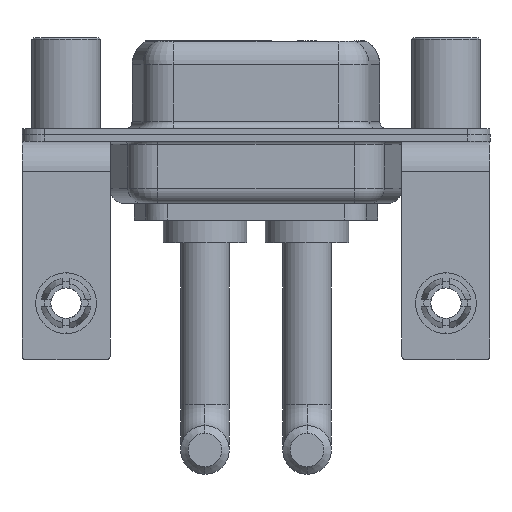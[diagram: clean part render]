
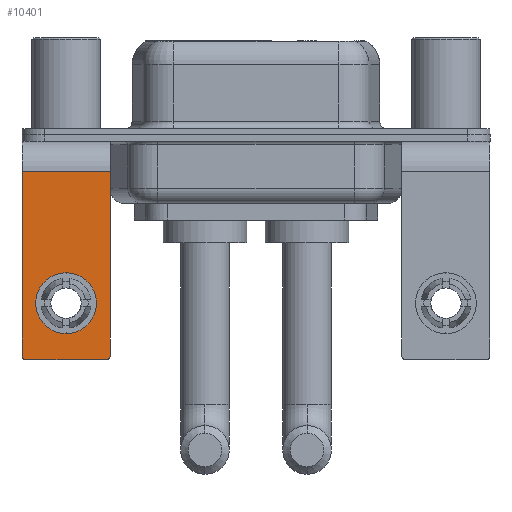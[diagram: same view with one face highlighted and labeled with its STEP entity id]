
A CAD part, front view. The second image highlights one B-rep face of the part: STEP entity #10401.
In plain terms, the highlighted planar face has unit normal (0, -1, 0).
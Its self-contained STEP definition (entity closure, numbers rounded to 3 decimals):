
#57 = CARTESIAN_POINT ( 'NONE',  ( 0., -6.25, -11.07 ) ) ;
#238 = DIRECTION ( 'NONE',  ( 0., 0., 1. ) ) ;
#415 = LINE ( 'NONE', #11838, #12715 ) ;
#627 = CARTESIAN_POINT ( 'NONE',  ( -2.9, -6.25, -2.4 ) ) ;
#634 = VERTEX_POINT ( 'NONE', #9744 ) ;
#840 = ORIENTED_EDGE ( 'NONE', *, *, #11025, .T. ) ;
#907 = VERTEX_POINT ( 'NONE', #14019 ) ;
#1452 = ORIENTED_EDGE ( 'NONE', *, *, #11088, .T. ) ;
#1684 = EDGE_CURVE ( 'NONE', #11396, #2459, #415, .T. ) ;
#1938 = VERTEX_POINT ( 'NONE', #7392 ) ;
#2459 = VERTEX_POINT ( 'NONE', #6097 ) ;
#3362 = CARTESIAN_POINT ( 'NONE',  ( -2.65, -6.25, -14.55 ) ) ;
#3517 = VECTOR ( 'NONE', #6561, 1000. ) ;
#3568 = LINE ( 'NONE', #8512, #11217 ) ;
#3751 = CARTESIAN_POINT ( 'NONE',  ( 2.9, -6.25, -14.8 ) ) ;
#3844 = EDGE_CURVE ( 'NONE', #8929, #10270, #5111, .T. ) ;
#3912 = DIRECTION ( 'NONE',  ( 0., 1., 0. ) ) ;
#3952 = CARTESIAN_POINT ( 'NONE',  ( 2.9, -6.25, -2.4 ) ) ;
#4049 = DIRECTION ( 'NONE',  ( 0., 0., 1. ) ) ;
#4340 = AXIS2_PLACEMENT_3D ( 'NONE', #5327, #14279, #4049 ) ;
#4439 = VERTEX_POINT ( 'NONE', #16140 ) ;
#4689 = AXIS2_PLACEMENT_3D ( 'NONE', #13130, #12094, #238 ) ;
#4721 = LINE ( 'NONE', #627, #5753 ) ;
#5111 = LINE ( 'NONE', #3751, #3517 ) ;
#5327 = CARTESIAN_POINT ( 'NONE',  ( 2.65, -6.25, -14.55 ) ) ;
#5480 = AXIS2_PLACEMENT_3D ( 'NONE', #3362, #13765, #10933 ) ;
#5485 = ORIENTED_EDGE ( 'NONE', *, *, #12165, .F. ) ;
#5627 = DIRECTION ( 'NONE',  ( -1., 0., 0. ) ) ;
#5642 = CARTESIAN_POINT ( 'NONE',  ( -2.65, -6.25, -14.8 ) ) ;
#5753 = VECTOR ( 'NONE', #14873, 1000. ) ;
#5783 = EDGE_LOOP ( 'NONE', ( #1452, #840, #5959, #12111, #5485, #14763 ) ) ;
#5956 = EDGE_CURVE ( 'NONE', #1938, #634, #7096, .T. ) ;
#5959 = ORIENTED_EDGE ( 'NONE', *, *, #3844, .F. ) ;
#6097 = CARTESIAN_POINT ( 'NONE',  ( -2.9, -6.25, -2.4 ) ) ;
#6231 = FACE_OUTER_BOUND ( 'NONE', #5783, .T. ) ;
#6299 = CIRCLE ( 'NONE', #5480, 0.25 ) ;
#6561 = DIRECTION ( 'NONE',  ( -1., 0., 0. ) ) ;
#7029 = CARTESIAN_POINT ( 'NONE',  ( 2.65, -6.25, -14.8 ) ) ;
#7096 = CIRCLE ( 'NONE', #16633, 2. ) ;
#7226 = ORIENTED_EDGE ( 'NONE', *, *, #13735, .T. ) ;
#7254 = DIRECTION ( 'NONE',  ( 0., 1., 0. ) ) ;
#7392 = CARTESIAN_POINT ( 'NONE',  ( 0., -6.25, -13.07 ) ) ;
#7878 = CIRCLE ( 'NONE', #4340, 0.25 ) ;
#8512 = CARTESIAN_POINT ( 'NONE',  ( 2.9, -6.25, -2.4 ) ) ;
#8772 = CIRCLE ( 'NONE', #4689, 2. ) ;
#8929 = VERTEX_POINT ( 'NONE', #7029 ) ;
#9444 = EDGE_LOOP ( 'NONE', ( #10554, #7226 ) ) ;
#9606 = EDGE_CURVE ( 'NONE', #8929, #4439, #7878, .T. ) ;
#9744 = CARTESIAN_POINT ( 'NONE',  ( 0., -6.25, -9.07 ) ) ;
#10270 = VERTEX_POINT ( 'NONE', #5642 ) ;
#10401 = ADVANCED_FACE ( 'NONE', ( #16711, #6231 ), #11512, .F. ) ;
#10554 = ORIENTED_EDGE ( 'NONE', *, *, #5956, .T. ) ;
#10933 = DIRECTION ( 'NONE',  ( 0., 0., 1. ) ) ;
#11025 = EDGE_CURVE ( 'NONE', #907, #10270, #6299, .T. ) ;
#11088 = EDGE_CURVE ( 'NONE', #2459, #907, #4721, .T. ) ;
#11217 = VECTOR ( 'NONE', #13724, 1000. ) ;
#11396 = VERTEX_POINT ( 'NONE', #3952 ) ;
#11512 = PLANE ( 'NONE',  #13078 ) ;
#11838 = CARTESIAN_POINT ( 'NONE',  ( 2.9, -6.25, -2.4 ) ) ;
#12094 = DIRECTION ( 'NONE',  ( 0., 1., 0. ) ) ;
#12111 = ORIENTED_EDGE ( 'NONE', *, *, #9606, .T. ) ;
#12165 = EDGE_CURVE ( 'NONE', #11396, #4439, #3568, .T. ) ;
#12540 = DIRECTION ( 'NONE',  ( 0., 0., 1. ) ) ;
#12715 = VECTOR ( 'NONE', #5627, 1000. ) ;
#12799 = CARTESIAN_POINT ( 'NONE',  ( 2.9, -6.25, -2.4 ) ) ;
#13078 = AXIS2_PLACEMENT_3D ( 'NONE', #12799, #7254, #12540 ) ;
#13130 = CARTESIAN_POINT ( 'NONE',  ( 0., -6.25, -11.07 ) ) ;
#13724 = DIRECTION ( 'NONE',  ( 0., 0., -1. ) ) ;
#13735 = EDGE_CURVE ( 'NONE', #634, #1938, #8772, .T. ) ;
#13765 = DIRECTION ( 'NONE',  ( 0., -1., 0. ) ) ;
#14019 = CARTESIAN_POINT ( 'NONE',  ( -2.9, -6.25, -14.55 ) ) ;
#14279 = DIRECTION ( 'NONE',  ( 0., -1., 0. ) ) ;
#14763 = ORIENTED_EDGE ( 'NONE', *, *, #1684, .T. ) ;
#14873 = DIRECTION ( 'NONE',  ( 0., 0., -1. ) ) ;
#15345 = DIRECTION ( 'NONE',  ( 0., 0., 1. ) ) ;
#16140 = CARTESIAN_POINT ( 'NONE',  ( 2.9, -6.25, -14.55 ) ) ;
#16633 = AXIS2_PLACEMENT_3D ( 'NONE', #57, #3912, #15345 ) ;
#16711 = FACE_BOUND ( 'NONE', #9444, .T. ) ;
